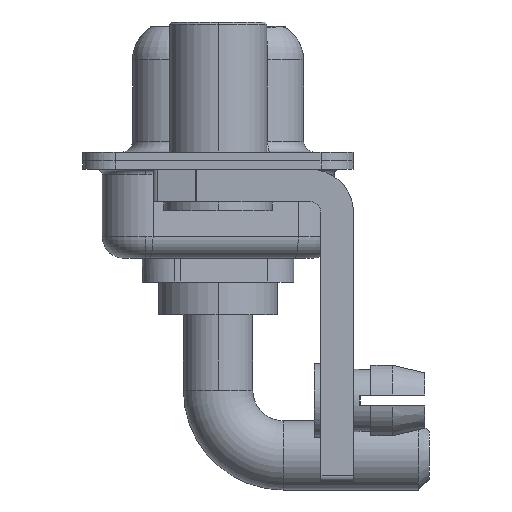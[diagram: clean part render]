
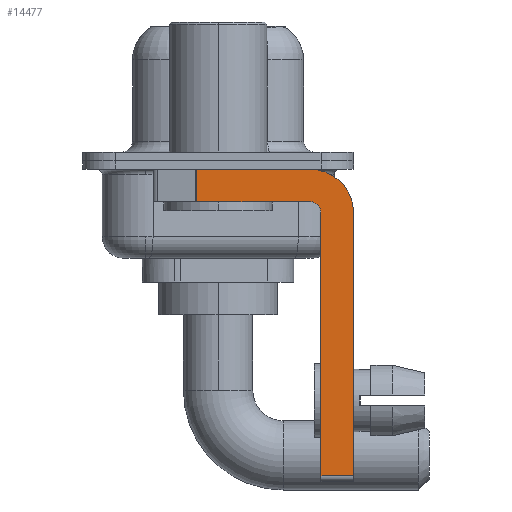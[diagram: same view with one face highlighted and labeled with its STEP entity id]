
A CAD part, left-side view. The second image highlights one B-rep face of the part: STEP entity #14477.
In plain terms, the highlighted planar face has unit normal (-1, 0, 0).
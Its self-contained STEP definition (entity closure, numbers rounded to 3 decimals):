
#129 = ORIENTED_EDGE ( 'NONE', *, *, #3534, .F. ) ;
#151 = AXIS2_PLACEMENT_3D ( 'NONE', #16375, #4963, #1430 ) ;
#161 = CARTESIAN_POINT ( 'NONE',  ( -2.9, 0.978, -1.9 ) ) ;
#460 = LINE ( 'NONE', #3973, #1226 ) ;
#556 = EDGE_CURVE ( 'NONE', #867, #8546, #13556, .T. ) ;
#867 = VERTEX_POINT ( 'NONE', #6773 ) ;
#1031 = VECTOR ( 'NONE', #4157, 1000. ) ;
#1226 = VECTOR ( 'NONE', #10454, 1000. ) ;
#1430 = DIRECTION ( 'NONE',  ( 0., 0., -1. ) ) ;
#1640 = LINE ( 'NONE', #14401, #1031 ) ;
#1920 = ORIENTED_EDGE ( 'NONE', *, *, #556, .T. ) ;
#2376 = VECTOR ( 'NONE', #13187, 1000. ) ;
#2826 = DIRECTION ( 'NONE',  ( 0., 0., 1. ) ) ;
#3014 = LINE ( 'NONE', #6764, #2376 ) ;
#3105 = ORIENTED_EDGE ( 'NONE', *, *, #10163, .F. ) ;
#3319 = CARTESIAN_POINT ( 'NONE',  ( -2.9, -4.75, -14.8 ) ) ;
#3534 = EDGE_CURVE ( 'NONE', #6742, #4454, #15599, .T. ) ;
#3812 = CARTESIAN_POINT ( 'NONE',  ( -2.9, -6.25, -2.4 ) ) ;
#3973 = CARTESIAN_POINT ( 'NONE',  ( -2.9, -6.25, -2.4 ) ) ;
#4157 = DIRECTION ( 'NONE',  ( 0., -1., 0. ) ) ;
#4273 = VECTOR ( 'NONE', #9670, 1000. ) ;
#4454 = VERTEX_POINT ( 'NONE', #3812 ) ;
#4503 = VERTEX_POINT ( 'NONE', #14219 ) ;
#4763 = CARTESIAN_POINT ( 'NONE',  ( -2.9, 3., -0.4 ) ) ;
#4812 = ORIENTED_EDGE ( 'NONE', *, *, #8272, .F. ) ;
#4815 = AXIS2_PLACEMENT_3D ( 'NONE', #12301, #10727, #2826 ) ;
#4871 = ORIENTED_EDGE ( 'NONE', *, *, #7262, .T. ) ;
#4963 = DIRECTION ( 'NONE',  ( 1., 0., 0. ) ) ;
#5392 = CARTESIAN_POINT ( 'NONE',  ( -2.9, -4.25, -0.4 ) ) ;
#5523 = CARTESIAN_POINT ( 'NONE',  ( -2.9, -6.25, -14.55 ) ) ;
#5889 = CARTESIAN_POINT ( 'NONE',  ( -2.9, 0.978, -1.9 ) ) ;
#5959 = EDGE_CURVE ( 'NONE', #4503, #10127, #14747, .T. ) ;
#6742 = VERTEX_POINT ( 'NONE', #5392 ) ;
#6764 = CARTESIAN_POINT ( 'NONE',  ( -2.9, -4.25, -1.9 ) ) ;
#6773 = CARTESIAN_POINT ( 'NONE',  ( -2.9, 0.978, -0.4 ) ) ;
#7262 = EDGE_CURVE ( 'NONE', #4503, #15707, #1640, .T. ) ;
#7416 = CARTESIAN_POINT ( 'NONE',  ( -2.9, -4.25, -2.4 ) ) ;
#8272 = EDGE_CURVE ( 'NONE', #10049, #8546, #3014, .T. ) ;
#8546 = VERTEX_POINT ( 'NONE', #161 ) ;
#8656 = EDGE_CURVE ( 'NONE', #10127, #10049, #8782, .T. ) ;
#8782 = CIRCLE ( 'NONE', #4815, 0.5 ) ;
#9441 = ORIENTED_EDGE ( 'NONE', *, *, #8656, .F. ) ;
#9670 = DIRECTION ( 'NONE',  ( 0., -1., 0. ) ) ;
#9916 = LINE ( 'NONE', #4763, #4273 ) ;
#10049 = VERTEX_POINT ( 'NONE', #13347 ) ;
#10127 = VERTEX_POINT ( 'NONE', #12003 ) ;
#10163 = EDGE_CURVE ( 'NONE', #867, #6742, #9916, .T. ) ;
#10454 = DIRECTION ( 'NONE',  ( 0., 0., -1. ) ) ;
#10727 = DIRECTION ( 'NONE',  ( -1., 0., 0. ) ) ;
#11245 = PLANE ( 'NONE',  #14010 ) ;
#11533 = ORIENTED_EDGE ( 'NONE', *, *, #14497, .F. ) ;
#11986 = ORIENTED_EDGE ( 'NONE', *, *, #5959, .F. ) ;
#12003 = CARTESIAN_POINT ( 'NONE',  ( -2.9, -4.75, -2.4 ) ) ;
#12175 = VECTOR ( 'NONE', #12399, 1000. ) ;
#12301 = CARTESIAN_POINT ( 'NONE',  ( -2.9, -4.25, -2.4 ) ) ;
#12399 = DIRECTION ( 'NONE',  ( 0., 0., 1. ) ) ;
#12706 = VECTOR ( 'NONE', #16045, 1000. ) ;
#13187 = DIRECTION ( 'NONE',  ( 0., 1., 0. ) ) ;
#13347 = CARTESIAN_POINT ( 'NONE',  ( -2.9, -4.25, -1.9 ) ) ;
#13504 = FACE_OUTER_BOUND ( 'NONE', #15726, .T. ) ;
#13556 = LINE ( 'NONE', #5889, #12706 ) ;
#13753 = DIRECTION ( 'NONE',  ( 1., 0., 0. ) ) ;
#14010 = AXIS2_PLACEMENT_3D ( 'NONE', #7416, #13753, #14752 ) ;
#14219 = CARTESIAN_POINT ( 'NONE',  ( -2.9, -4.75, -14.55 ) ) ;
#14401 = CARTESIAN_POINT ( 'NONE',  ( -2.9, -4.25, -14.55 ) ) ;
#14477 = ADVANCED_FACE ( 'NONE', ( #13504 ), #11245, .F. ) ;
#14497 = EDGE_CURVE ( 'NONE', #4454, #15707, #460, .T. ) ;
#14747 = LINE ( 'NONE', #3319, #12175 ) ;
#14752 = DIRECTION ( 'NONE',  ( 0., 0., -1. ) ) ;
#15599 = CIRCLE ( 'NONE', #151, 2. ) ;
#15707 = VERTEX_POINT ( 'NONE', #5523 ) ;
#15726 = EDGE_LOOP ( 'NONE', ( #3105, #1920, #4812, #9441, #11986, #4871, #11533, #129 ) ) ;
#16045 = DIRECTION ( 'NONE',  ( 0., 0., -1. ) ) ;
#16375 = CARTESIAN_POINT ( 'NONE',  ( -2.9, -4.25, -2.4 ) ) ;
